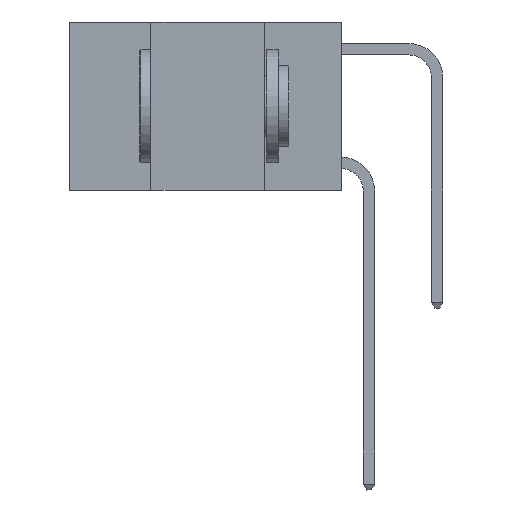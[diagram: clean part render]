
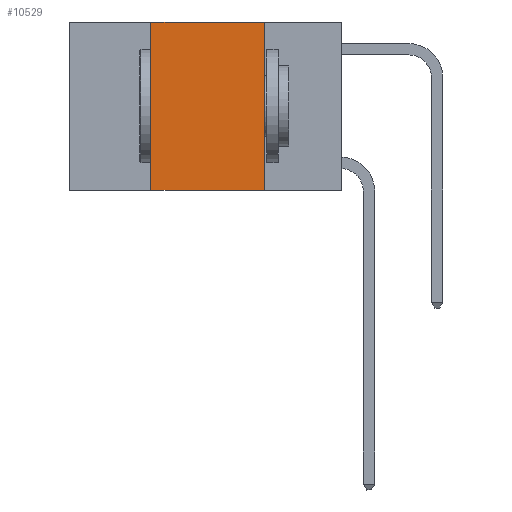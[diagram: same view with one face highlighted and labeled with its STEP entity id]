
A CAD part, left-side view. The second image highlights one B-rep face of the part: STEP entity #10529.
In plain terms, the highlighted planar face has unit normal (-1, 0, 0).
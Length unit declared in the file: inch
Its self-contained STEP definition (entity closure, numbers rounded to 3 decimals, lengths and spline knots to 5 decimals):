
#736 = VERTEX_POINT ( 'NONE', #6036 ) ;
#1218 = VERTEX_POINT ( 'NONE', #18275 ) ;
#1509 = ORIENTED_EDGE ( 'NONE', *, *, #11357, .F. ) ;
#1512 = CARTESIAN_POINT ( 'NONE',  ( 0., 0.17, 0. ) ) ;
#1793 = EDGE_CURVE ( 'NONE', #4590, #1218, #8401, .T. ) ;
#3008 = EDGE_CURVE ( 'NONE', #21742, #736, #16399, .T. ) ;
#3149 = CARTESIAN_POINT ( 'NONE',  ( 0., 0.6, -0.37 ) ) ;
#4405 = CARTESIAN_POINT ( 'NONE',  ( 0., 0.6, 0. ) ) ;
#4590 = VERTEX_POINT ( 'NONE', #18709 ) ;
#4600 = DIRECTION ( 'NONE',  ( 0., 0., 1. ) ) ;
#4710 = CARTESIAN_POINT ( 'NONE',  ( 0., 0.42, 0. ) ) ;
#6036 = CARTESIAN_POINT ( 'NONE',  ( 0., 0.17, 0. ) ) ;
#6544 = DIRECTION ( 'NONE',  ( 0., 0., -1. ) ) ;
#6920 = AXIS2_PLACEMENT_3D ( 'NONE', #18210, #21930, #11310 ) ;
#7862 = DIRECTION ( 'NONE',  ( 0., -1., 0. ) ) ;
#8138 = FACE_OUTER_BOUND ( 'NONE', #14889, .T. ) ;
#8229 = LINE ( 'NONE', #1512, #17607 ) ;
#8401 = LINE ( 'NONE', #3149, #13943 ) ;
#10529 = ADVANCED_FACE ( 'NONE', ( #8138 ), #14980, .F. ) ;
#10637 = ORIENTED_EDGE ( 'NONE', *, *, #3008, .F. ) ;
#11310 = DIRECTION ( 'NONE',  ( 0., 0., -1. ) ) ;
#11357 = EDGE_CURVE ( 'NONE', #4590, #21742, #11552, .T. ) ;
#11552 = LINE ( 'NONE', #4710, #16268 ) ;
#11808 = VECTOR ( 'NONE', #7862, 39.37008 ) ;
#13943 = VECTOR ( 'NONE', #15251, 39.37008 ) ;
#14889 = EDGE_LOOP ( 'NONE', ( #19468, #10637, #1509, #20284 ) ) ;
#14980 = PLANE ( 'NONE',  #6920 ) ;
#15251 = DIRECTION ( 'NONE',  ( 0., -1., 0. ) ) ;
#16268 = VECTOR ( 'NONE', #4600, 39.37008 ) ;
#16399 = LINE ( 'NONE', #4405, #11808 ) ;
#17607 = VECTOR ( 'NONE', #6544, 39.37008 ) ;
#18210 = CARTESIAN_POINT ( 'NONE',  ( 0., 0.6, 0. ) ) ;
#18275 = CARTESIAN_POINT ( 'NONE',  ( 0., 0.17, -0.37 ) ) ;
#18709 = CARTESIAN_POINT ( 'NONE',  ( 0., 0.42, -0.37 ) ) ;
#19468 = ORIENTED_EDGE ( 'NONE', *, *, #20954, .F. ) ;
#19706 = CARTESIAN_POINT ( 'NONE',  ( 0., 0.42, 0. ) ) ;
#20284 = ORIENTED_EDGE ( 'NONE', *, *, #1793, .T. ) ;
#20954 = EDGE_CURVE ( 'NONE', #736, #1218, #8229, .T. ) ;
#21742 = VERTEX_POINT ( 'NONE', #19706 ) ;
#21930 = DIRECTION ( 'NONE',  ( 1., 0., 0. ) ) ;
